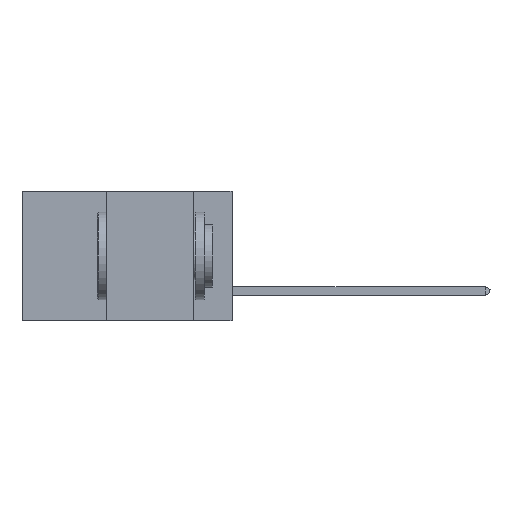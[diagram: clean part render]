
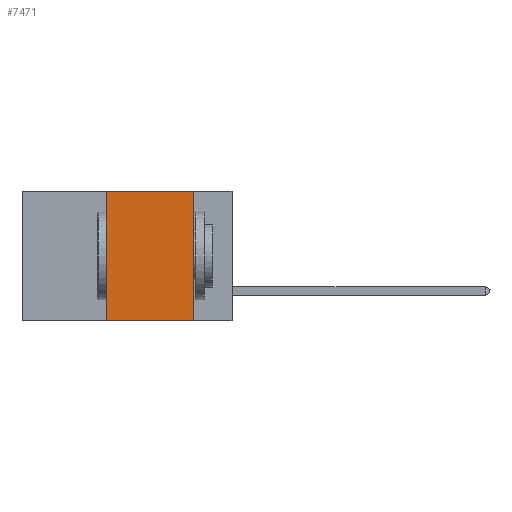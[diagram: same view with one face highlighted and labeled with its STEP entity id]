
A CAD part, left-side view. The second image highlights one B-rep face of the part: STEP entity #7471.
In plain terms, the highlighted planar face has unit normal (-1, 0, 0).
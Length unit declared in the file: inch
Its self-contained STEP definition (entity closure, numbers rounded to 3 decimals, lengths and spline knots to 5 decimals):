
#94 = CARTESIAN_POINT ( 'NONE',  ( 0., 0.6, 0. ) ) ;
#474 = ORIENTED_EDGE ( 'NONE', *, *, #5466, .T. ) ;
#710 = EDGE_CURVE ( 'NONE', #5684, #2055, #7361, .T. ) ;
#1129 = DIRECTION ( 'NONE',  ( 0., -1., 0. ) ) ;
#1143 = EDGE_CURVE ( 'NONE', #8095, #5684, #4233, .T. ) ;
#1318 = CARTESIAN_POINT ( 'NONE',  ( 0., 0.36, -0.37 ) ) ;
#1375 = VECTOR ( 'NONE', #1129, 39.37008 ) ;
#1401 = ORIENTED_EDGE ( 'NONE', *, *, #9155, .F. ) ;
#1559 = DIRECTION ( 'NONE',  ( 0., 0., 1. ) ) ;
#1655 = VECTOR ( 'NONE', #2508, 39.37008 ) ;
#1798 = CARTESIAN_POINT ( 'NONE',  ( 0., 0.11, 0. ) ) ;
#2055 = VERTEX_POINT ( 'NONE', #9015 ) ;
#2388 = LINE ( 'NONE', #1798, #1655 ) ;
#2508 = DIRECTION ( 'NONE',  ( 0., 0., -1. ) ) ;
#2692 = DIRECTION ( 'NONE',  ( 0., -1., 0. ) ) ;
#3311 = DIRECTION ( 'NONE',  ( 0., 0., -1. ) ) ;
#3471 = CARTESIAN_POINT ( 'NONE',  ( 0., 0.6, -0.37 ) ) ;
#3905 = CARTESIAN_POINT ( 'NONE',  ( 0., 0.36, 0. ) ) ;
#4123 = AXIS2_PLACEMENT_3D ( 'NONE', #94, #7894, #3311 ) ;
#4233 = LINE ( 'NONE', #3905, #5431 ) ;
#5217 = PLANE ( 'NONE',  #4123 ) ;
#5276 = VERTEX_POINT ( 'NONE', #6452 ) ;
#5431 = VECTOR ( 'NONE', #1559, 39.37008 ) ;
#5466 = EDGE_CURVE ( 'NONE', #8095, #5276, #5836, .T. ) ;
#5684 = VERTEX_POINT ( 'NONE', #6050 ) ;
#5836 = LINE ( 'NONE', #3471, #1375 ) ;
#6050 = CARTESIAN_POINT ( 'NONE',  ( 0., 0.36, 0. ) ) ;
#6189 = ORIENTED_EDGE ( 'NONE', *, *, #710, .F. ) ;
#6452 = CARTESIAN_POINT ( 'NONE',  ( 0., 0.11, -0.37 ) ) ;
#7208 = ORIENTED_EDGE ( 'NONE', *, *, #1143, .F. ) ;
#7361 = LINE ( 'NONE', #9570, #8808 ) ;
#7471 = ADVANCED_FACE ( 'NONE', ( #7613 ), #5217, .F. ) ;
#7613 = FACE_OUTER_BOUND ( 'NONE', #8691, .T. ) ;
#7894 = DIRECTION ( 'NONE',  ( 1., 0., 0. ) ) ;
#8095 = VERTEX_POINT ( 'NONE', #1318 ) ;
#8691 = EDGE_LOOP ( 'NONE', ( #1401, #6189, #7208, #474 ) ) ;
#8808 = VECTOR ( 'NONE', #2692, 39.37008 ) ;
#9015 = CARTESIAN_POINT ( 'NONE',  ( 0., 0.11, 0. ) ) ;
#9155 = EDGE_CURVE ( 'NONE', #2055, #5276, #2388, .T. ) ;
#9570 = CARTESIAN_POINT ( 'NONE',  ( 0., 0.6, 0. ) ) ;
